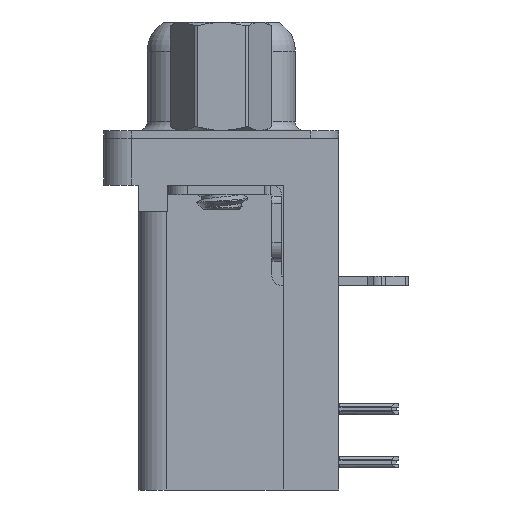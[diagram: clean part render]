
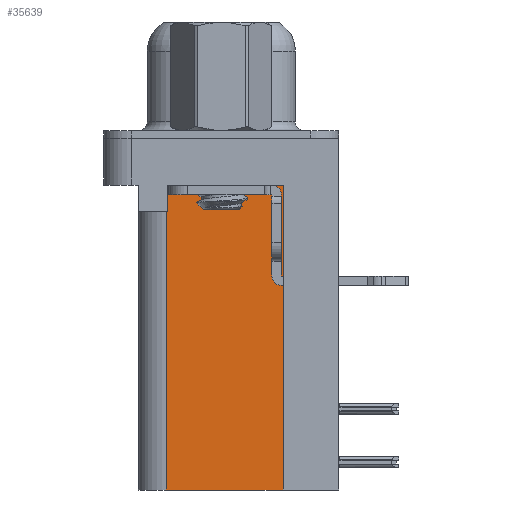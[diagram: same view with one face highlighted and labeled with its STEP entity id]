
A CAD part, left-side view. The second image highlights one B-rep face of the part: STEP entity #35639.
In plain terms, the highlighted planar face has unit normal (-1, 0, 0).
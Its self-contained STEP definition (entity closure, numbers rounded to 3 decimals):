
#195 = CARTESIAN_POINT ( 'NONE',  ( 3.79, -3.295, -18.76 ) ) ;
#1202 = EDGE_CURVE ( 'NONE', #10446, #31465, #17736, .T. ) ;
#3485 = EDGE_CURVE ( 'NONE', #13842, #15176, #18760, .T. ) ;
#3516 = LINE ( 'NONE', #36445, #11365 ) ;
#3811 = VECTOR ( 'NONE', #34444, 1000. ) ;
#4247 = CARTESIAN_POINT ( 'NONE',  ( 3.79, -3.295, -18.76 ) ) ;
#5243 = PLANE ( 'NONE',  #23936 ) ;
#5491 = EDGE_CURVE ( 'NONE', #13842, #28039, #30389, .T. ) ;
#5601 = EDGE_CURVE ( 'NONE', #28039, #10446, #11654, .T. ) ;
#8204 = DIRECTION ( 'NONE',  ( 1., 0., 0. ) ) ;
#8290 = DIRECTION ( 'NONE',  ( 0., 1., 0. ) ) ;
#10446 = VERTEX_POINT ( 'NONE', #31625 ) ;
#11365 = VECTOR ( 'NONE', #21497, 1000. ) ;
#11636 = FACE_OUTER_BOUND ( 'NONE', #29906, .T. ) ;
#11654 = LINE ( 'NONE', #22451, #3811 ) ;
#11737 = CARTESIAN_POINT ( 'NONE',  ( 3.79, -3.295, -18.76 ) ) ;
#13410 = CARTESIAN_POINT ( 'NONE',  ( 3.79, 2.925, -3.9 ) ) ;
#13585 = ORIENTED_EDGE ( 'NONE', *, *, #3485, .F. ) ;
#13842 = VERTEX_POINT ( 'NONE', #11737 ) ;
#14860 = ORIENTED_EDGE ( 'NONE', *, *, #1202, .T. ) ;
#15176 = VERTEX_POINT ( 'NONE', #30150 ) ;
#16192 = DIRECTION ( 'NONE',  ( 0., 0., -1. ) ) ;
#16463 = ORIENTED_EDGE ( 'NONE', *, *, #26121, .F. ) ;
#16808 = VECTOR ( 'NONE', #16192, 1000. ) ;
#17736 = LINE ( 'NONE', #35135, #16808 ) ;
#17769 = VECTOR ( 'NONE', #36004, 1000. ) ;
#18074 = CARTESIAN_POINT ( 'NONE',  ( 3.79, 2.925, -18.76 ) ) ;
#18137 = ORIENTED_EDGE ( 'NONE', *, *, #33441, .T. ) ;
#18760 = LINE ( 'NONE', #195, #25776 ) ;
#19659 = CARTESIAN_POINT ( 'NONE',  ( 3.79, 2.895, -3.9 ) ) ;
#21497 = DIRECTION ( 'NONE',  ( 0., 1., 0. ) ) ;
#21953 = DIRECTION ( 'NONE',  ( 0., 0., 1. ) ) ;
#22451 = CARTESIAN_POINT ( 'NONE',  ( 3.79, -3.295, -2.5 ) ) ;
#23248 = ORIENTED_EDGE ( 'NONE', *, *, #5491, .T. ) ;
#23936 = AXIS2_PLACEMENT_3D ( 'NONE', #25985, #8204, #29028 ) ;
#25776 = VECTOR ( 'NONE', #8290, 1000. ) ;
#25985 = CARTESIAN_POINT ( 'NONE',  ( 3.79, -3.295, -18.76 ) ) ;
#26121 = EDGE_CURVE ( 'NONE', #15176, #30063, #34650, .T. ) ;
#28039 = VERTEX_POINT ( 'NONE', #31457 ) ;
#29028 = DIRECTION ( 'NONE',  ( 0., 1., 0. ) ) ;
#29435 = VECTOR ( 'NONE', #21953, 1000. ) ;
#29906 = EDGE_LOOP ( 'NONE', ( #34958, #14860, #18137, #16463, #13585, #23248 ) ) ;
#30063 = VERTEX_POINT ( 'NONE', #13410 ) ;
#30150 = CARTESIAN_POINT ( 'NONE',  ( 3.79, 2.925, -18.76 ) ) ;
#30389 = LINE ( 'NONE', #4247, #29435 ) ;
#31457 = CARTESIAN_POINT ( 'NONE',  ( 3.79, -3.295, -2.5 ) ) ;
#31465 = VERTEX_POINT ( 'NONE', #19659 ) ;
#31625 = CARTESIAN_POINT ( 'NONE',  ( 3.79, 2.895, -2.5 ) ) ;
#33441 = EDGE_CURVE ( 'NONE', #31465, #30063, #3516, .T. ) ;
#34444 = DIRECTION ( 'NONE',  ( 0., 1., 0. ) ) ;
#34650 = LINE ( 'NONE', #18074, #17769 ) ;
#34958 = ORIENTED_EDGE ( 'NONE', *, *, #5601, .T. ) ;
#35135 = CARTESIAN_POINT ( 'NONE',  ( 3.79, 2.895, -3.9 ) ) ;
#35639 = ADVANCED_FACE ( 'NONE', ( #11636 ), #5243, .F. ) ;
#36004 = DIRECTION ( 'NONE',  ( 0., 0., 1. ) ) ;
#36445 = CARTESIAN_POINT ( 'NONE',  ( 3.79, 0., -3.9 ) ) ;
